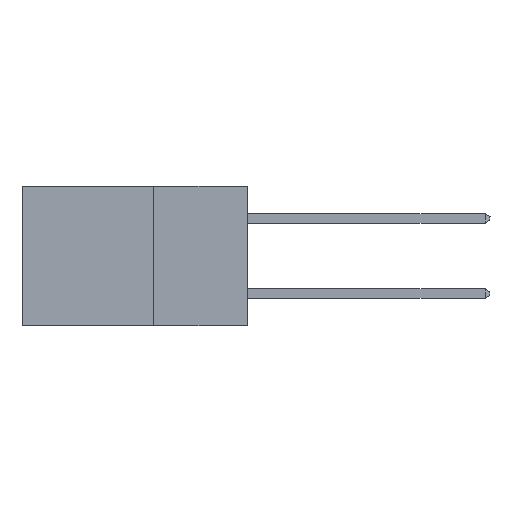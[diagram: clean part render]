
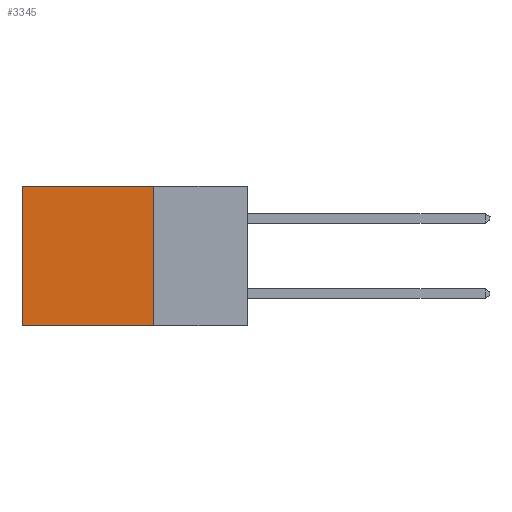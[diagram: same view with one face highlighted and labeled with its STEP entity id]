
A CAD part, left-side view. The second image highlights one B-rep face of the part: STEP entity #3345.
In plain terms, the highlighted planar face has unit normal (-1, 0, 0).
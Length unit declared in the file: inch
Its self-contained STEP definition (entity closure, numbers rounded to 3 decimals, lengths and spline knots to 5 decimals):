
#243 = LINE ( 'NONE', #4185, #10713 ) ;
#323 = LINE ( 'NONE', #13147, #8493 ) ;
#340 = ORIENTED_EDGE ( 'NONE', *, *, #3214, .F. ) ;
#379 = DIRECTION ( 'NONE',  ( 1., 0., 0. ) ) ;
#749 = AXIS2_PLACEMENT_3D ( 'NONE', #7783, #379, #1554 ) ;
#1554 = DIRECTION ( 'NONE',  ( 0., 0., -1. ) ) ;
#1635 = VECTOR ( 'NONE', #10926, 39.37008 ) ;
#1661 = DIRECTION ( 'NONE',  ( 0., 0., -1. ) ) ;
#2285 = CARTESIAN_POINT ( 'NONE',  ( 0.2615, 0.25, -0.37 ) ) ;
#2597 = DIRECTION ( 'NONE',  ( 0., 1., 0. ) ) ;
#3214 = EDGE_CURVE ( 'NONE', #6026, #10060, #243, .T. ) ;
#3345 = ADVANCED_FACE ( 'NONE', ( #9879 ), #9031, .F. ) ;
#4165 = ORIENTED_EDGE ( 'NONE', *, *, #10263, .F. ) ;
#4185 = CARTESIAN_POINT ( 'NONE',  ( 0.2615, 0.25, -0.37 ) ) ;
#4303 = VERTEX_POINT ( 'NONE', #13181 ) ;
#4688 = VECTOR ( 'NONE', #1661, 39.37008 ) ;
#5180 = CARTESIAN_POINT ( 'NONE',  ( 0.2615, 0.25, 0. ) ) ;
#5214 = CARTESIAN_POINT ( 'NONE',  ( 0.2615, 0.6, -0.37 ) ) ;
#6026 = VERTEX_POINT ( 'NONE', #12057 ) ;
#6575 = EDGE_CURVE ( 'NONE', #13650, #4303, #323, .T. ) ;
#6682 = CARTESIAN_POINT ( 'NONE',  ( 0.2615, 0.6, -0.37 ) ) ;
#7783 = CARTESIAN_POINT ( 'NONE',  ( 0.2615, 0.25, -0.37 ) ) ;
#7908 = EDGE_CURVE ( 'NONE', #4303, #10060, #9948, .T. ) ;
#8124 = ORIENTED_EDGE ( 'NONE', *, *, #7908, .T. ) ;
#8493 = VECTOR ( 'NONE', #2597, 39.37008 ) ;
#8694 = DIRECTION ( 'NONE',  ( 0., 1., 0. ) ) ;
#9031 = PLANE ( 'NONE',  #749 ) ;
#9446 = ORIENTED_EDGE ( 'NONE', *, *, #6575, .T. ) ;
#9879 = FACE_OUTER_BOUND ( 'NONE', #11767, .T. ) ;
#9948 = LINE ( 'NONE', #6682, #1635 ) ;
#10060 = VERTEX_POINT ( 'NONE', #5214 ) ;
#10263 = EDGE_CURVE ( 'NONE', #13650, #6026, #11794, .T. ) ;
#10713 = VECTOR ( 'NONE', #8694, 39.37008 ) ;
#10926 = DIRECTION ( 'NONE',  ( 0., 0., -1. ) ) ;
#11767 = EDGE_LOOP ( 'NONE', ( #8124, #340, #4165, #9446 ) ) ;
#11794 = LINE ( 'NONE', #2285, #4688 ) ;
#12057 = CARTESIAN_POINT ( 'NONE',  ( 0.2615, 0.25, -0.37 ) ) ;
#13147 = CARTESIAN_POINT ( 'NONE',  ( 0.2615, 0.25, 0. ) ) ;
#13181 = CARTESIAN_POINT ( 'NONE',  ( 0.2615, 0.6, 0. ) ) ;
#13650 = VERTEX_POINT ( 'NONE', #5180 ) ;
